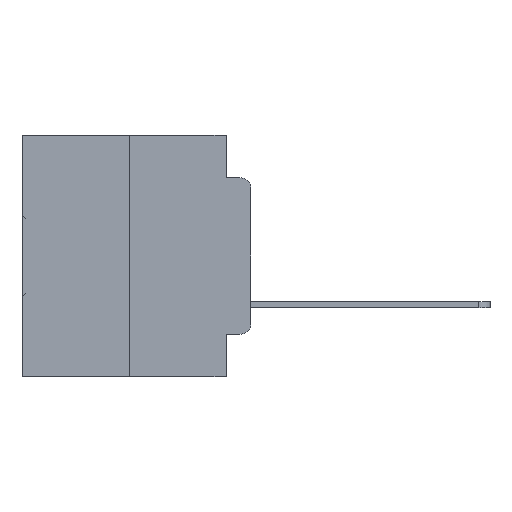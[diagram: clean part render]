
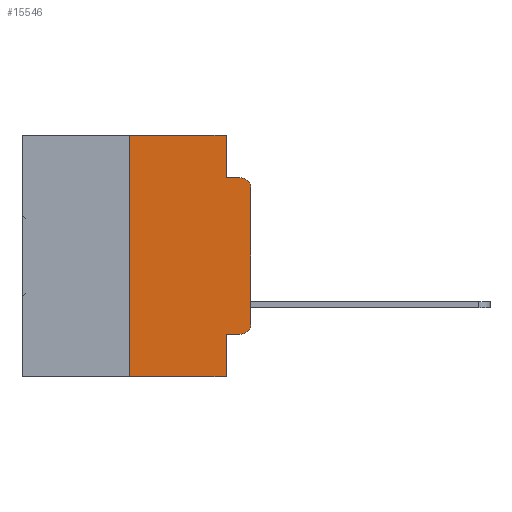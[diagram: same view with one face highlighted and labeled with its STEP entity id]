
A CAD part, left-side view. The second image highlights one B-rep face of the part: STEP entity #15546.
In plain terms, the highlighted planar face has unit normal (-1, 0, 0).
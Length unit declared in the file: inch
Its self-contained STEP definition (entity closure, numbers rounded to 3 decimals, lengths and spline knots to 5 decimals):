
#415 = ORIENTED_EDGE ( 'NONE', *, *, #23078, .F. ) ;
#1174 = EDGE_CURVE ( 'NONE', #17513, #27086, #28839, .T. ) ;
#1454 = VERTEX_POINT ( 'NONE', #4515 ) ;
#1530 = VECTOR ( 'NONE', #18351, 39.37008 ) ;
#2046 = LINE ( 'NONE', #28400, #30926 ) ;
#2152 = DIRECTION ( 'NONE',  ( 0., -1., 0. ) ) ;
#2197 = LINE ( 'NONE', #10591, #27506 ) ;
#2467 = EDGE_CURVE ( 'NONE', #27325, #1454, #7941, .T. ) ;
#2941 = VERTEX_POINT ( 'NONE', #14484 ) ;
#4454 = DIRECTION ( 'NONE',  ( 0., 0., -1. ) ) ;
#4515 = CARTESIAN_POINT ( 'NONE',  ( 0., 0.02, -0.0885 ) ) ;
#5335 = PLANE ( 'NONE',  #11414 ) ;
#5662 = EDGE_CURVE ( 'NONE', #14501, #27325, #19614, .T. ) ;
#6341 = ORIENTED_EDGE ( 'NONE', *, *, #17017, .T. ) ;
#7197 = CARTESIAN_POINT ( 'NONE',  ( 0., 0.051, -0.4115 ) ) ;
#7562 = DIRECTION ( 'NONE',  ( -1., 0., 0. ) ) ;
#7786 = FACE_OUTER_BOUND ( 'NONE', #29014, .T. ) ;
#7941 = CIRCLE ( 'NONE', #12432, 0.02 ) ;
#8133 = DIRECTION ( 'NONE',  ( 1., 0., 0. ) ) ;
#8394 = CARTESIAN_POINT ( 'NONE',  ( 0., 0.02, -0.1085 ) ) ;
#9260 = CARTESIAN_POINT ( 'NONE',  ( 0., 0.051, -0.5 ) ) ;
#9784 = CARTESIAN_POINT ( 'NONE',  ( 0., 0., -0.1085 ) ) ;
#10415 = ORIENTED_EDGE ( 'NONE', *, *, #25872, .F. ) ;
#10591 = CARTESIAN_POINT ( 'NONE',  ( 0., 0.051, 0. ) ) ;
#11414 = AXIS2_PLACEMENT_3D ( 'NONE', #32044, #8133, #31541 ) ;
#11979 = CARTESIAN_POINT ( 'NONE',  ( 0., 0., 0. ) ) ;
#12179 = VERTEX_POINT ( 'NONE', #32968 ) ;
#12432 = AXIS2_PLACEMENT_3D ( 'NONE', #8394, #19038, #29699 ) ;
#12811 = DIRECTION ( 'NONE',  ( 0., -1., 0. ) ) ;
#13427 = DIRECTION ( 'NONE',  ( 0., 0., 1. ) ) ;
#13976 = VECTOR ( 'NONE', #12811, 39.37008 ) ;
#14069 = ORIENTED_EDGE ( 'NONE', *, *, #5662, .T. ) ;
#14484 = CARTESIAN_POINT ( 'NONE',  ( 0., 0.051, -0.0885 ) ) ;
#14501 = VERTEX_POINT ( 'NONE', #25205 ) ;
#14614 = CARTESIAN_POINT ( 'NONE',  ( 0., 0.02, -0.3915 ) ) ;
#14627 = DIRECTION ( 'NONE',  ( 0., -1., 0. ) ) ;
#14808 = CARTESIAN_POINT ( 'NONE',  ( 0., 0.051, -0.0885 ) ) ;
#15546 = ADVANCED_FACE ( 'NONE', ( #7786 ), #5335, .F. ) ;
#16107 = CARTESIAN_POINT ( 'NONE',  ( 0., 0.473, -0.5 ) ) ;
#16736 = AXIS2_PLACEMENT_3D ( 'NONE', #14614, #7562, #30660 ) ;
#17017 = EDGE_CURVE ( 'NONE', #26909, #12179, #30953, .T. ) ;
#17221 = CARTESIAN_POINT ( 'NONE',  ( 0., 0.051, 0. ) ) ;
#17513 = VERTEX_POINT ( 'NONE', #17776 ) ;
#17571 = VECTOR ( 'NONE', #13427, 39.37008 ) ;
#17776 = CARTESIAN_POINT ( 'NONE',  ( 0., 0.25, -0.5 ) ) ;
#17848 = VERTEX_POINT ( 'NONE', #17221 ) ;
#18229 = CARTESIAN_POINT ( 'NONE',  ( 0., 0.473, 0. ) ) ;
#18351 = DIRECTION ( 'NONE',  ( 0., 0., 1. ) ) ;
#19027 = VECTOR ( 'NONE', #34434, 39.37008 ) ;
#19038 = DIRECTION ( 'NONE',  ( -1., 0., 0. ) ) ;
#19614 = LINE ( 'NONE', #11979, #17571 ) ;
#19917 = VECTOR ( 'NONE', #14627, 39.37008 ) ;
#20272 = CARTESIAN_POINT ( 'NONE',  ( 0., 0.25, 0. ) ) ;
#21208 = ORIENTED_EDGE ( 'NONE', *, *, #25535, .F. ) ;
#22079 = ORIENTED_EDGE ( 'NONE', *, *, #2467, .T. ) ;
#22353 = ORIENTED_EDGE ( 'NONE', *, *, #1174, .T. ) ;
#23078 = EDGE_CURVE ( 'NONE', #26909, #27086, #2046, .T. ) ;
#24154 = ORIENTED_EDGE ( 'NONE', *, *, #30568, .F. ) ;
#24463 = ORIENTED_EDGE ( 'NONE', *, *, #33842, .F. ) ;
#25205 = CARTESIAN_POINT ( 'NONE',  ( 0., 0., -0.3915 ) ) ;
#25535 = EDGE_CURVE ( 'NONE', #17513, #25536, #33736, .T. ) ;
#25536 = VERTEX_POINT ( 'NONE', #20272 ) ;
#25872 = EDGE_CURVE ( 'NONE', #2941, #1454, #33300, .T. ) ;
#25972 = DIRECTION ( 'NONE',  ( 0., 0., -1. ) ) ;
#26081 = LINE ( 'NONE', #18229, #33000 ) ;
#26723 = CARTESIAN_POINT ( 'NONE',  ( 0., 0.051, -0.4115 ) ) ;
#26909 = VERTEX_POINT ( 'NONE', #26723 ) ;
#27086 = VERTEX_POINT ( 'NONE', #9260 ) ;
#27325 = VERTEX_POINT ( 'NONE', #9784 ) ;
#27506 = VECTOR ( 'NONE', #4454, 39.37008 ) ;
#28400 = CARTESIAN_POINT ( 'NONE',  ( 0., 0.051, 0. ) ) ;
#28806 = EDGE_CURVE ( 'NONE', #12179, #14501, #31776, .T. ) ;
#28839 = LINE ( 'NONE', #16107, #19027 ) ;
#29014 = EDGE_LOOP ( 'NONE', ( #14069, #22079, #10415, #24463, #24154, #21208, #22353, #415, #6341, #32862 ) ) ;
#29699 = DIRECTION ( 'NONE',  ( 0., 0., -1. ) ) ;
#30568 = EDGE_CURVE ( 'NONE', #25536, #17848, #26081, .T. ) ;
#30660 = DIRECTION ( 'NONE',  ( 0., 0., -1. ) ) ;
#30926 = VECTOR ( 'NONE', #25972, 39.37008 ) ;
#30953 = LINE ( 'NONE', #7197, #13976 ) ;
#31447 = CARTESIAN_POINT ( 'NONE',  ( 0., 0.25, 0. ) ) ;
#31541 = DIRECTION ( 'NONE',  ( 0., 0., -1. ) ) ;
#31776 = CIRCLE ( 'NONE', #16736, 0.02 ) ;
#32044 = CARTESIAN_POINT ( 'NONE',  ( 0., 0.473, 0. ) ) ;
#32862 = ORIENTED_EDGE ( 'NONE', *, *, #28806, .T. ) ;
#32968 = CARTESIAN_POINT ( 'NONE',  ( 0., 0.02, -0.4115 ) ) ;
#33000 = VECTOR ( 'NONE', #2152, 39.37008 ) ;
#33300 = LINE ( 'NONE', #14808, #19917 ) ;
#33736 = LINE ( 'NONE', #31447, #1530 ) ;
#33842 = EDGE_CURVE ( 'NONE', #17848, #2941, #2197, .T. ) ;
#34434 = DIRECTION ( 'NONE',  ( 0., -1., 0. ) ) ;
